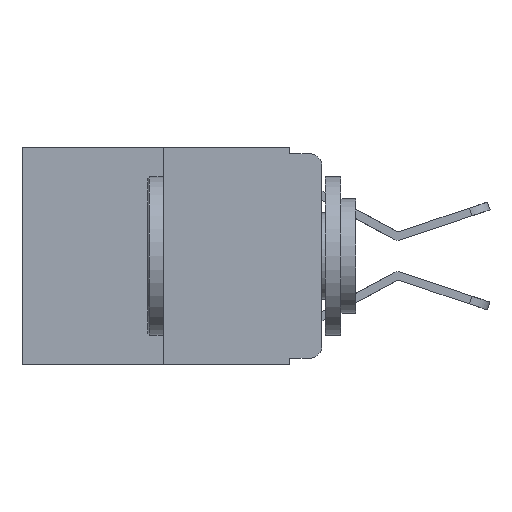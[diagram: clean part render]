
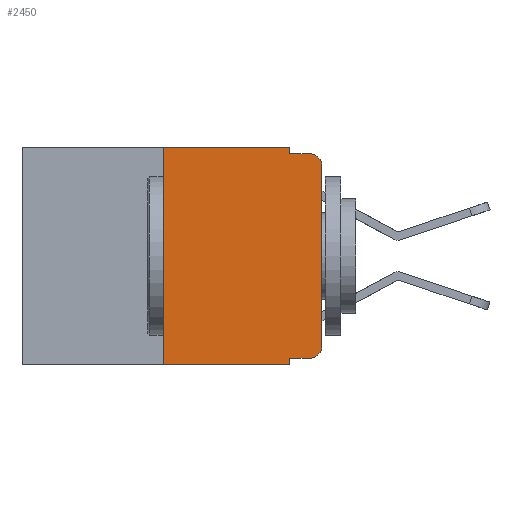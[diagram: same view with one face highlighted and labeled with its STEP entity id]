
A CAD part, left-side view. The second image highlights one B-rep face of the part: STEP entity #2450.
In plain terms, the highlighted planar face has unit normal (-1, 0, 0).
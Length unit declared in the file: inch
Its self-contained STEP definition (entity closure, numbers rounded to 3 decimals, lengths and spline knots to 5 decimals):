
#78 = EDGE_CURVE ( 'NONE', #3097, #7855, #9220, .T. ) ;
#235 = EDGE_CURVE ( 'NONE', #4781, #11320, #11347, .T. ) ;
#280 = VERTEX_POINT ( 'NONE', #686 ) ;
#425 = CARTESIAN_POINT ( 'NONE',  ( 0., 0.25, -0.343 ) ) ;
#559 = VECTOR ( 'NONE', #4038, 39.37008 ) ;
#686 = CARTESIAN_POINT ( 'NONE',  ( 0., 0.02, -0.333 ) ) ;
#721 = VERTEX_POINT ( 'NONE', #1757 ) ;
#914 = DIRECTION ( 'NONE',  ( -1., 0., 0. ) ) ;
#985 = VECTOR ( 'NONE', #2140, 39.37008 ) ;
#1024 = EDGE_CURVE ( 'NONE', #10384, #6455, #9616, .T. ) ;
#1030 = CARTESIAN_POINT ( 'NONE',  ( 0., 0.25, 0. ) ) ;
#1069 = CARTESIAN_POINT ( 'NONE',  ( 0., 0.473, 0. ) ) ;
#1148 = ORIENTED_EDGE ( 'NONE', *, *, #7365, .T. ) ;
#1233 = AXIS2_PLACEMENT_3D ( 'NONE', #6384, #5685, #1525 ) ;
#1357 = DIRECTION ( 'NONE',  ( 0., 0., -1. ) ) ;
#1360 = ORIENTED_EDGE ( 'NONE', *, *, #8029, .T. ) ;
#1525 = DIRECTION ( 'NONE',  ( 0., 0., -1. ) ) ;
#1646 = CARTESIAN_POINT ( 'NONE',  ( 0., 0.051, 0. ) ) ;
#1750 = CARTESIAN_POINT ( 'NONE',  ( 0., 0., -0.03 ) ) ;
#1757 = CARTESIAN_POINT ( 'NONE',  ( 0., 0., -0.313 ) ) ;
#1810 = DIRECTION ( 'NONE',  ( 0., 0., -1. ) ) ;
#1870 = ORIENTED_EDGE ( 'NONE', *, *, #1024, .F. ) ;
#2072 = CARTESIAN_POINT ( 'NONE',  ( 0., 0.25, 0. ) ) ;
#2140 = DIRECTION ( 'NONE',  ( 0., 0., -1. ) ) ;
#2174 = LINE ( 'NONE', #5845, #9716 ) ;
#2216 = AXIS2_PLACEMENT_3D ( 'NONE', #6096, #914, #1357 ) ;
#2369 = EDGE_CURVE ( 'NONE', #7544, #6455, #5822, .T. ) ;
#2378 = DIRECTION ( 'NONE',  ( 0., -1., 0. ) ) ;
#2450 = ADVANCED_FACE ( 'NONE', ( #11390 ), #4689, .F. ) ;
#2479 = EDGE_LOOP ( 'NONE', ( #10957, #11591, #4431, #10187, #4345, #7223, #7637, #1870, #1360, #1148 ) ) ;
#2660 = DIRECTION ( 'NONE',  ( 0., -1., 0. ) ) ;
#3097 = VERTEX_POINT ( 'NONE', #1750 ) ;
#3204 = CIRCLE ( 'NONE', #9177, 0.02 ) ;
#3257 = LINE ( 'NONE', #1030, #559 ) ;
#3379 = VECTOR ( 'NONE', #2660, 39.37008 ) ;
#3418 = CARTESIAN_POINT ( 'NONE',  ( 0., 0.051, -0.343 ) ) ;
#3967 = LINE ( 'NONE', #10463, #8452 ) ;
#4038 = DIRECTION ( 'NONE',  ( 0., 0., 1. ) ) ;
#4170 = DIRECTION ( 'NONE',  ( 0., 0., -1. ) ) ;
#4345 = ORIENTED_EDGE ( 'NONE', *, *, #235, .F. ) ;
#4431 = ORIENTED_EDGE ( 'NONE', *, *, #11810, .F. ) ;
#4668 = VECTOR ( 'NONE', #1810, 39.37008 ) ;
#4689 = PLANE ( 'NONE',  #1233 ) ;
#4692 = VECTOR ( 'NONE', #10832, 39.37008 ) ;
#4733 = VERTEX_POINT ( 'NONE', #9048 ) ;
#4781 = VERTEX_POINT ( 'NONE', #2072 ) ;
#5255 = LINE ( 'NONE', #6839, #985 ) ;
#5333 = VECTOR ( 'NONE', #2378, 39.37008 ) ;
#5685 = DIRECTION ( 'NONE',  ( 1., 0., 0. ) ) ;
#5804 = DIRECTION ( 'NONE',  ( 0., -1., 0. ) ) ;
#5822 = LINE ( 'NONE', #6011, #3379 ) ;
#5845 = CARTESIAN_POINT ( 'NONE',  ( 0., 0.051, -0.333 ) ) ;
#6011 = CARTESIAN_POINT ( 'NONE',  ( 0., 0.473, -0.343 ) ) ;
#6096 = CARTESIAN_POINT ( 'NONE',  ( 0., 0.02, -0.03 ) ) ;
#6118 = CARTESIAN_POINT ( 'NONE',  ( 0., 0.051, -0.01 ) ) ;
#6384 = CARTESIAN_POINT ( 'NONE',  ( 0., 0.473, 0. ) ) ;
#6408 = CARTESIAN_POINT ( 'NONE',  ( 0., 0.02, -0.01 ) ) ;
#6455 = VERTEX_POINT ( 'NONE', #3418 ) ;
#6839 = CARTESIAN_POINT ( 'NONE',  ( 0., 0.051, 0. ) ) ;
#7223 = ORIENTED_EDGE ( 'NONE', *, *, #8660, .F. ) ;
#7365 = EDGE_CURVE ( 'NONE', #280, #721, #3204, .T. ) ;
#7544 = VERTEX_POINT ( 'NONE', #425 ) ;
#7637 = ORIENTED_EDGE ( 'NONE', *, *, #2369, .T. ) ;
#7700 = LINE ( 'NONE', #6118, #5333 ) ;
#7855 = VERTEX_POINT ( 'NONE', #6408 ) ;
#8029 = EDGE_CURVE ( 'NONE', #10384, #280, #2174, .T. ) ;
#8126 = CARTESIAN_POINT ( 'NONE',  ( 0., 0.02, -0.313 ) ) ;
#8452 = VECTOR ( 'NONE', #11319, 39.37008 ) ;
#8660 = EDGE_CURVE ( 'NONE', #7544, #4781, #3257, .T. ) ;
#9048 = CARTESIAN_POINT ( 'NONE',  ( 0., 0.051, -0.01 ) ) ;
#9090 = CARTESIAN_POINT ( 'NONE',  ( 0., 0.051, 0. ) ) ;
#9177 = AXIS2_PLACEMENT_3D ( 'NONE', #8126, #9473, #4170 ) ;
#9220 = CIRCLE ( 'NONE', #2216, 0.02 ) ;
#9473 = DIRECTION ( 'NONE',  ( -1., 0., 0. ) ) ;
#9616 = LINE ( 'NONE', #9090, #4668 ) ;
#9716 = VECTOR ( 'NONE', #5804, 39.37008 ) ;
#10187 = ORIENTED_EDGE ( 'NONE', *, *, #11008, .F. ) ;
#10361 = CARTESIAN_POINT ( 'NONE',  ( 0., 0.051, -0.333 ) ) ;
#10384 = VERTEX_POINT ( 'NONE', #10361 ) ;
#10463 = CARTESIAN_POINT ( 'NONE',  ( 0., 0., 0. ) ) ;
#10832 = DIRECTION ( 'NONE',  ( 0., -1., 0. ) ) ;
#10957 = ORIENTED_EDGE ( 'NONE', *, *, #11105, .T. ) ;
#11008 = EDGE_CURVE ( 'NONE', #11320, #4733, #5255, .T. ) ;
#11105 = EDGE_CURVE ( 'NONE', #721, #3097, #3967, .T. ) ;
#11319 = DIRECTION ( 'NONE',  ( 0., 0., 1. ) ) ;
#11320 = VERTEX_POINT ( 'NONE', #1646 ) ;
#11347 = LINE ( 'NONE', #1069, #4692 ) ;
#11390 = FACE_OUTER_BOUND ( 'NONE', #2479, .T. ) ;
#11591 = ORIENTED_EDGE ( 'NONE', *, *, #78, .T. ) ;
#11810 = EDGE_CURVE ( 'NONE', #4733, #7855, #7700, .T. ) ;
